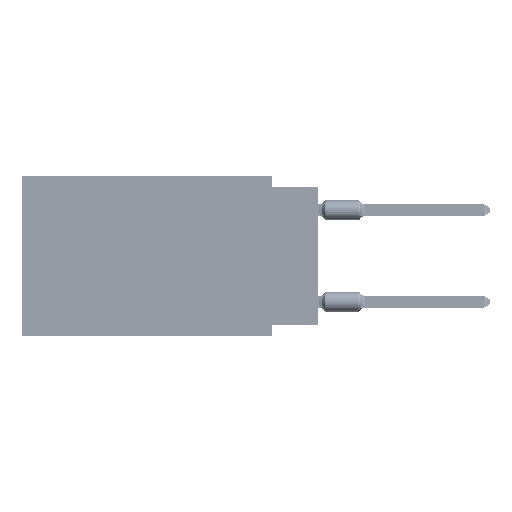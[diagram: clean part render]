
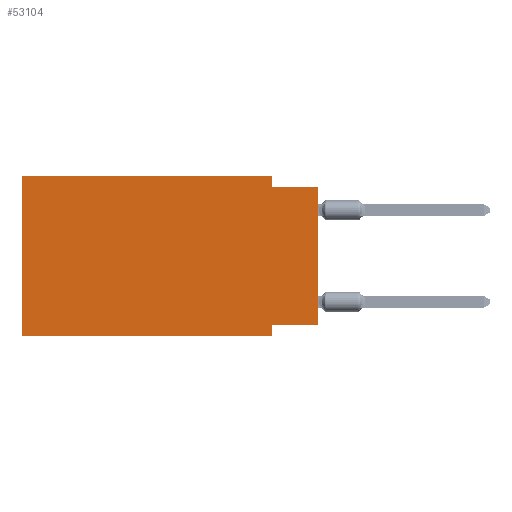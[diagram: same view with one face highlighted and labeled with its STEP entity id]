
A CAD part, left-side view. The second image highlights one B-rep face of the part: STEP entity #53104.
In plain terms, the highlighted planar face has unit normal (-1, 0, 0).
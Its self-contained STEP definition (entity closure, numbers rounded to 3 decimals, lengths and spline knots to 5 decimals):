
#1135 = VECTOR ( 'NONE', #17712, 39.37008 ) ;
#1807 = CARTESIAN_POINT ( 'NONE',  ( 0., 0., -0.325 ) ) ;
#3670 = VECTOR ( 'NONE', #72686, 39.37008 ) ;
#10222 = DIRECTION ( 'NONE',  ( 0., -1., 0. ) ) ;
#11695 = LINE ( 'NONE', #26776, #50141 ) ;
#13184 = EDGE_CURVE ( 'NONE', #56924, #44103, #27968, .T. ) ;
#14207 = LINE ( 'NONE', #22273, #98813 ) ;
#14884 = EDGE_CURVE ( 'NONE', #50661, #90636, #11695, .T. ) ;
#15822 = VERTEX_POINT ( 'NONE', #79196 ) ;
#16313 = CARTESIAN_POINT ( 'NONE',  ( 0., 0.1, -0.325 ) ) ;
#16326 = EDGE_CURVE ( 'NONE', #73293, #56924, #47421, .T. ) ;
#17193 = LINE ( 'NONE', #58080, #1135 ) ;
#17712 = DIRECTION ( 'NONE',  ( 0., -1., 0. ) ) ;
#20379 = CARTESIAN_POINT ( 'NONE',  ( 0., 0.1, -0.35 ) ) ;
#22273 = CARTESIAN_POINT ( 'NONE',  ( 0., 0.1, -0.35 ) ) ;
#22589 = VECTOR ( 'NONE', #75264, 39.37008 ) ;
#26776 = CARTESIAN_POINT ( 'NONE',  ( 0., 0., -0.325 ) ) ;
#27968 = LINE ( 'NONE', #37094, #97977 ) ;
#33583 = EDGE_CURVE ( 'NONE', #73293, #97902, #17193, .T. ) ;
#37094 = CARTESIAN_POINT ( 'NONE',  ( 0., 0.645, 0. ) ) ;
#38595 = CARTESIAN_POINT ( 'NONE',  ( 0., 0.645, 0. ) ) ;
#40944 = ORIENTED_EDGE ( 'NONE', *, *, #90673, .F. ) ;
#41417 = CARTESIAN_POINT ( 'NONE',  ( 0., 0., -0.025 ) ) ;
#42604 = LINE ( 'NONE', #74348, #88810 ) ;
#43586 = EDGE_CURVE ( 'NONE', #44103, #15822, #42604, .T. ) ;
#44103 = VERTEX_POINT ( 'NONE', #68255 ) ;
#44492 = DIRECTION ( 'NONE',  ( 0., 1., 0. ) ) ;
#46125 = FACE_OUTER_BOUND ( 'NONE', #66909, .T. ) ;
#47421 = LINE ( 'NONE', #65147, #3670 ) ;
#50141 = VECTOR ( 'NONE', #44492, 39.37008 ) ;
#50661 = VERTEX_POINT ( 'NONE', #1807 ) ;
#51279 = ORIENTED_EDGE ( 'NONE', *, *, #16326, .F. ) ;
#53071 = ORIENTED_EDGE ( 'NONE', *, *, #76756, .T. ) ;
#53104 = ADVANCED_FACE ( 'NONE', ( #46125 ), #79992, .F. ) ;
#53974 = ORIENTED_EDGE ( 'NONE', *, *, #13184, .F. ) ;
#55091 = DIRECTION ( 'NONE',  ( 0., 0., -1. ) ) ;
#56924 = VERTEX_POINT ( 'NONE', #94389 ) ;
#58080 = CARTESIAN_POINT ( 'NONE',  ( 0., 0.645, -0.35 ) ) ;
#58775 = LINE ( 'NONE', #68415, #105418 ) ;
#65147 = CARTESIAN_POINT ( 'NONE',  ( 0., 0.645, 0. ) ) ;
#65645 = AXIS2_PLACEMENT_3D ( 'NONE', #38595, #104191, #96152 ) ;
#66909 = EDGE_LOOP ( 'NONE', ( #53071, #76847, #71582, #53974, #51279, #81268, #40944, #69469 ) ) ;
#67483 = CARTESIAN_POINT ( 'NONE',  ( 0., 0.645, -0.35 ) ) ;
#68255 = CARTESIAN_POINT ( 'NONE',  ( 0., 0.1, 0. ) ) ;
#68415 = CARTESIAN_POINT ( 'NONE',  ( 0., 0., 0. ) ) ;
#69469 = ORIENTED_EDGE ( 'NONE', *, *, #14884, .F. ) ;
#71582 = ORIENTED_EDGE ( 'NONE', *, *, #43586, .F. ) ;
#72686 = DIRECTION ( 'NONE',  ( 0., 0., 1. ) ) ;
#73293 = VERTEX_POINT ( 'NONE', #67483 ) ;
#74348 = CARTESIAN_POINT ( 'NONE',  ( 0., 0.1, 0. ) ) ;
#75264 = DIRECTION ( 'NONE',  ( 0., -1., 0. ) ) ;
#76489 = DIRECTION ( 'NONE',  ( 0., 0., 1. ) ) ;
#76756 = EDGE_CURVE ( 'NONE', #50661, #93032, #58775, .T. ) ;
#76847 = ORIENTED_EDGE ( 'NONE', *, *, #84096, .F. ) ;
#79196 = CARTESIAN_POINT ( 'NONE',  ( 0., 0.1, -0.025 ) ) ;
#79992 = PLANE ( 'NONE',  #65645 ) ;
#81268 = ORIENTED_EDGE ( 'NONE', *, *, #33583, .T. ) ;
#81365 = CARTESIAN_POINT ( 'NONE',  ( 0., 0., -0.025 ) ) ;
#84096 = EDGE_CURVE ( 'NONE', #15822, #93032, #92479, .T. ) ;
#88810 = VECTOR ( 'NONE', #100138, 39.37008 ) ;
#90636 = VERTEX_POINT ( 'NONE', #16313 ) ;
#90673 = EDGE_CURVE ( 'NONE', #90636, #97902, #14207, .T. ) ;
#92479 = LINE ( 'NONE', #41417, #22589 ) ;
#93032 = VERTEX_POINT ( 'NONE', #81365 ) ;
#94389 = CARTESIAN_POINT ( 'NONE',  ( 0., 0.645, 0. ) ) ;
#96152 = DIRECTION ( 'NONE',  ( 0., 0., -1. ) ) ;
#97902 = VERTEX_POINT ( 'NONE', #20379 ) ;
#97977 = VECTOR ( 'NONE', #10222, 39.37008 ) ;
#98813 = VECTOR ( 'NONE', #55091, 39.37008 ) ;
#100138 = DIRECTION ( 'NONE',  ( 0., 0., -1. ) ) ;
#104191 = DIRECTION ( 'NONE',  ( 1., 0., 0. ) ) ;
#105418 = VECTOR ( 'NONE', #76489, 39.37008 ) ;
